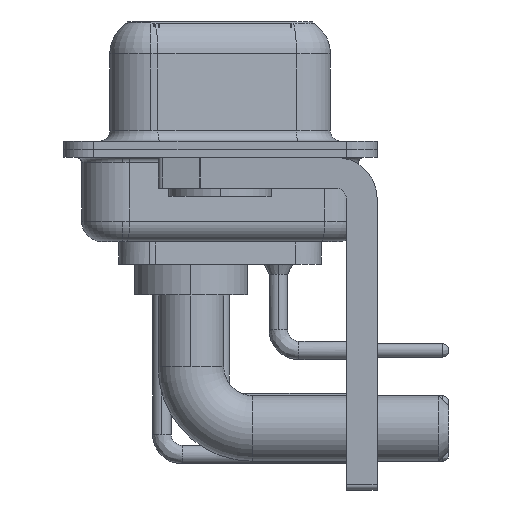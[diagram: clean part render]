
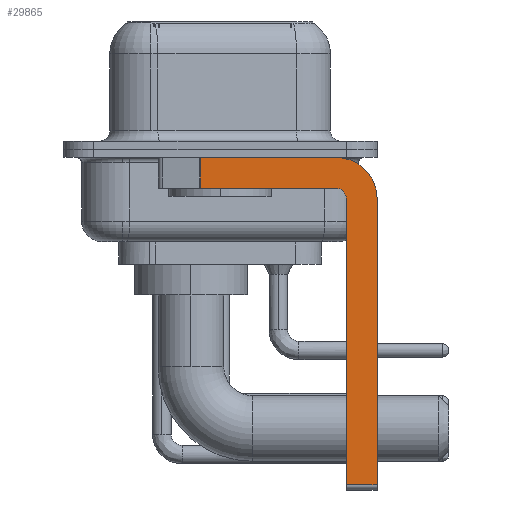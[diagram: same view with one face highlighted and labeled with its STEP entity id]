
A CAD part, left-side view. The second image highlights one B-rep face of the part: STEP entity #29865.
In plain terms, the highlighted planar face has unit normal (-1, 0, 0).
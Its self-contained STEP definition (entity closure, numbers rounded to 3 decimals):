
#569 = CARTESIAN_POINT ( 'NONE',  ( -2.9, -5.65, -1.9 ) ) ;
#953 = CARTESIAN_POINT ( 'NONE',  ( -2.9, 0.978, -1.9 ) ) ;
#1064 = CARTESIAN_POINT ( 'NONE',  ( -2.9, -7.65, -2.4 ) ) ;
#1275 = EDGE_LOOP ( 'NONE', ( #16029, #24164, #26084, #6301, #26093, #29580, #10095, #13644 ) ) ;
#2119 = CARTESIAN_POINT ( 'NONE',  ( -2.9, -5.65, -16.35 ) ) ;
#2470 = LINE ( 'NONE', #2119, #28519 ) ;
#2555 = DIRECTION ( 'NONE',  ( 0., 0., 1. ) ) ;
#2642 = CARTESIAN_POINT ( 'NONE',  ( -2.9, -7.65, -2.4 ) ) ;
#2829 = CARTESIAN_POINT ( 'NONE',  ( -2.9, -5.65, -2.4 ) ) ;
#3200 = LINE ( 'NONE', #569, #7726 ) ;
#3383 = CARTESIAN_POINT ( 'NONE',  ( -2.9, -7.65, -16.35 ) ) ;
#3743 = VECTOR ( 'NONE', #4239, 1000. ) ;
#4045 = VERTEX_POINT ( 'NONE', #17488 ) ;
#4239 = DIRECTION ( 'NONE',  ( 0., 0., -1. ) ) ;
#5018 = CIRCLE ( 'NONE', #11750, 0.5 ) ;
#5463 = FACE_OUTER_BOUND ( 'NONE', #1275, .T. ) ;
#5843 = EDGE_CURVE ( 'NONE', #28522, #21354, #5018, .T. ) ;
#6119 = CIRCLE ( 'NONE', #25750, 2. ) ;
#6194 = DIRECTION ( 'NONE',  ( -1., 0., 0. ) ) ;
#6301 = ORIENTED_EDGE ( 'NONE', *, *, #5843, .F. ) ;
#6429 = CARTESIAN_POINT ( 'NONE',  ( -2.9, 3., -0.4 ) ) ;
#6810 = DIRECTION ( 'NONE',  ( 0., 0., -1. ) ) ;
#6895 = DIRECTION ( 'NONE',  ( 0., 0., 1. ) ) ;
#7726 = VECTOR ( 'NONE', #11311, 1000. ) ;
#7858 = EDGE_CURVE ( 'NONE', #4045, #28522, #26522, .T. ) ;
#9513 = EDGE_CURVE ( 'NONE', #21971, #15628, #31996, .T. ) ;
#9873 = LINE ( 'NONE', #17794, #3743 ) ;
#10095 = ORIENTED_EDGE ( 'NONE', *, *, #9513, .F. ) ;
#11311 = DIRECTION ( 'NONE',  ( 0., 1., 0. ) ) ;
#11750 = AXIS2_PLACEMENT_3D ( 'NONE', #26470, #6194, #2555 ) ;
#12074 = DIRECTION ( 'NONE',  ( 0., -1., 0. ) ) ;
#13028 = CARTESIAN_POINT ( 'NONE',  ( -2.9, -6.15, -16.6 ) ) ;
#13401 = EDGE_CURVE ( 'NONE', #13934, #15919, #30336, .T. ) ;
#13583 = DIRECTION ( 'NONE',  ( 1., 0., 0. ) ) ;
#13644 = ORIENTED_EDGE ( 'NONE', *, *, #23744, .F. ) ;
#13934 = VERTEX_POINT ( 'NONE', #15162 ) ;
#14053 = CARTESIAN_POINT ( 'NONE',  ( -2.9, -5.65, -0.4 ) ) ;
#14103 = EDGE_CURVE ( 'NONE', #4045, #15628, #2470, .T. ) ;
#15162 = CARTESIAN_POINT ( 'NONE',  ( -2.9, 0.978, -0.4 ) ) ;
#15628 = VERTEX_POINT ( 'NONE', #3383 ) ;
#15919 = VERTEX_POINT ( 'NONE', #14053 ) ;
#16029 = ORIENTED_EDGE ( 'NONE', *, *, #13401, .F. ) ;
#16204 = PLANE ( 'NONE',  #21640 ) ;
#16711 = DIRECTION ( 'NONE',  ( 0., 0., -1. ) ) ;
#17012 = CARTESIAN_POINT ( 'NONE',  ( -2.9, -6.15, -2.4 ) ) ;
#17488 = CARTESIAN_POINT ( 'NONE',  ( -2.9, -6.15, -16.35 ) ) ;
#17794 = CARTESIAN_POINT ( 'NONE',  ( -2.9, 0.978, -1.9 ) ) ;
#20271 = VECTOR ( 'NONE', #16711, 1000. ) ;
#21354 = VERTEX_POINT ( 'NONE', #24680 ) ;
#21640 = AXIS2_PLACEMENT_3D ( 'NONE', #2829, #13583, #24277 ) ;
#21971 = VERTEX_POINT ( 'NONE', #1064 ) ;
#23744 = EDGE_CURVE ( 'NONE', #15919, #21971, #6119, .T. ) ;
#24099 = DIRECTION ( 'NONE',  ( 0., -1., 0. ) ) ;
#24164 = ORIENTED_EDGE ( 'NONE', *, *, #30768, .T. ) ;
#24277 = DIRECTION ( 'NONE',  ( 0., 0., -1. ) ) ;
#24680 = CARTESIAN_POINT ( 'NONE',  ( -2.9, -5.65, -1.9 ) ) ;
#25750 = AXIS2_PLACEMENT_3D ( 'NONE', #33847, #30882, #6810 ) ;
#26084 = ORIENTED_EDGE ( 'NONE', *, *, #32231, .F. ) ;
#26093 = ORIENTED_EDGE ( 'NONE', *, *, #7858, .F. ) ;
#26470 = CARTESIAN_POINT ( 'NONE',  ( -2.9, -5.65, -2.4 ) ) ;
#26522 = LINE ( 'NONE', #13028, #32068 ) ;
#28519 = VECTOR ( 'NONE', #24099, 1000. ) ;
#28522 = VERTEX_POINT ( 'NONE', #17012 ) ;
#28920 = VERTEX_POINT ( 'NONE', #953 ) ;
#29580 = ORIENTED_EDGE ( 'NONE', *, *, #14103, .T. ) ;
#29806 = VECTOR ( 'NONE', #12074, 1000. ) ;
#29865 = ADVANCED_FACE ( 'NONE', ( #5463 ), #16204, .F. ) ;
#30336 = LINE ( 'NONE', #6429, #29806 ) ;
#30768 = EDGE_CURVE ( 'NONE', #13934, #28920, #9873, .T. ) ;
#30882 = DIRECTION ( 'NONE',  ( 1., 0., 0. ) ) ;
#31996 = LINE ( 'NONE', #2642, #20271 ) ;
#32068 = VECTOR ( 'NONE', #6895, 1000. ) ;
#32231 = EDGE_CURVE ( 'NONE', #21354, #28920, #3200, .T. ) ;
#33847 = CARTESIAN_POINT ( 'NONE',  ( -2.9, -5.65, -2.4 ) ) ;
